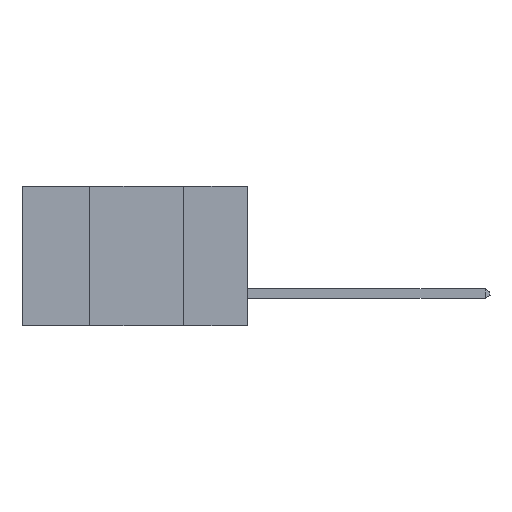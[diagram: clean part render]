
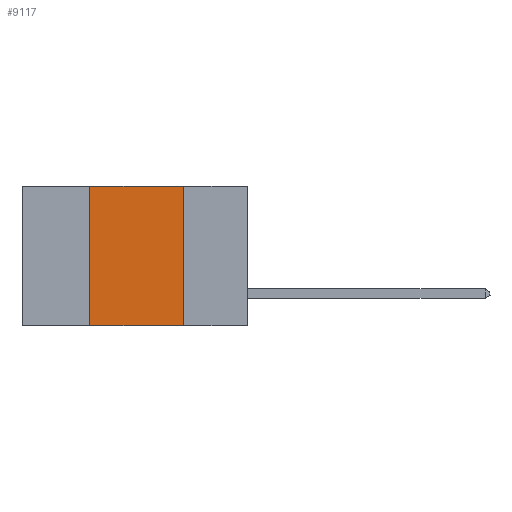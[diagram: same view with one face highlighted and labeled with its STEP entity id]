
A CAD part, left-side view. The second image highlights one B-rep face of the part: STEP entity #9117.
In plain terms, the highlighted planar face has unit normal (-1, 0, 0).
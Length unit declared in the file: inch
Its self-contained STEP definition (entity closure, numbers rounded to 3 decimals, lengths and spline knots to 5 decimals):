
#23 = VERTEX_POINT ( 'NONE', #686 ) ;
#618 = CARTESIAN_POINT ( 'NONE',  ( 0., 0.6, -0.37 ) ) ;
#686 = CARTESIAN_POINT ( 'NONE',  ( 0., 0.17, 0. ) ) ;
#794 = CARTESIAN_POINT ( 'NONE',  ( 0., 0.17, 0. ) ) ;
#810 = VERTEX_POINT ( 'NONE', #4985 ) ;
#1051 = FACE_OUTER_BOUND ( 'NONE', #3674, .T. ) ;
#1116 = CARTESIAN_POINT ( 'NONE',  ( 0., 0.6, 0. ) ) ;
#1227 = EDGE_CURVE ( 'NONE', #11543, #810, #12173, .T. ) ;
#1268 = LINE ( 'NONE', #794, #5951 ) ;
#1588 = EDGE_CURVE ( 'NONE', #11543, #12572, #12481, .T. ) ;
#2792 = AXIS2_PLACEMENT_3D ( 'NONE', #9392, #9256, #6402 ) ;
#2915 = LINE ( 'NONE', #1116, #4611 ) ;
#3674 = EDGE_LOOP ( 'NONE', ( #9006, #5786, #5795, #8274 ) ) ;
#4611 = VECTOR ( 'NONE', #8098, 39.37008 ) ;
#4985 = CARTESIAN_POINT ( 'NONE',  ( 0., 0.42, 0. ) ) ;
#5423 = PLANE ( 'NONE',  #2792 ) ;
#5786 = ORIENTED_EDGE ( 'NONE', *, *, #9632, .F. ) ;
#5795 = ORIENTED_EDGE ( 'NONE', *, *, #1227, .F. ) ;
#5951 = VECTOR ( 'NONE', #12583, 39.37008 ) ;
#6402 = DIRECTION ( 'NONE',  ( 0., 0., -1. ) ) ;
#6851 = EDGE_CURVE ( 'NONE', #23, #12572, #1268, .T. ) ;
#6889 = VECTOR ( 'NONE', #9181, 39.37008 ) ;
#8098 = DIRECTION ( 'NONE',  ( 0., -1., 0. ) ) ;
#8256 = CARTESIAN_POINT ( 'NONE',  ( 0., 0.42, 0. ) ) ;
#8274 = ORIENTED_EDGE ( 'NONE', *, *, #1588, .T. ) ;
#8668 = CARTESIAN_POINT ( 'NONE',  ( 0., 0.17, -0.37 ) ) ;
#9006 = ORIENTED_EDGE ( 'NONE', *, *, #6851, .F. ) ;
#9117 = ADVANCED_FACE ( 'NONE', ( #1051 ), #5423, .F. ) ;
#9181 = DIRECTION ( 'NONE',  ( 0., 0., 1. ) ) ;
#9256 = DIRECTION ( 'NONE',  ( 1., 0., 0. ) ) ;
#9392 = CARTESIAN_POINT ( 'NONE',  ( 0., 0.6, 0. ) ) ;
#9632 = EDGE_CURVE ( 'NONE', #810, #23, #2915, .T. ) ;
#9678 = DIRECTION ( 'NONE',  ( 0., -1., 0. ) ) ;
#11543 = VERTEX_POINT ( 'NONE', #12050 ) ;
#12023 = VECTOR ( 'NONE', #9678, 39.37008 ) ;
#12050 = CARTESIAN_POINT ( 'NONE',  ( 0., 0.42, -0.37 ) ) ;
#12173 = LINE ( 'NONE', #8256, #6889 ) ;
#12481 = LINE ( 'NONE', #618, #12023 ) ;
#12572 = VERTEX_POINT ( 'NONE', #8668 ) ;
#12583 = DIRECTION ( 'NONE',  ( 0., 0., -1. ) ) ;
